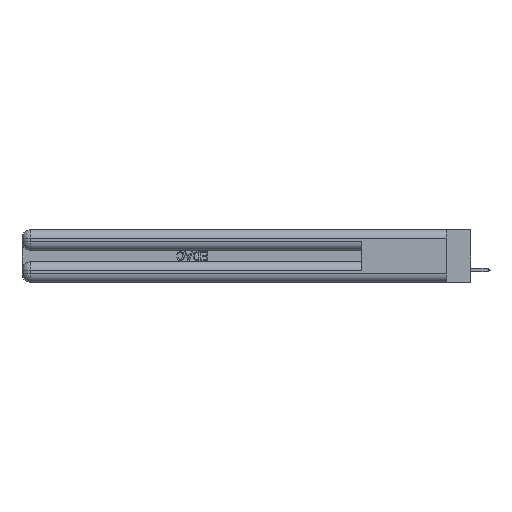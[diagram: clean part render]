
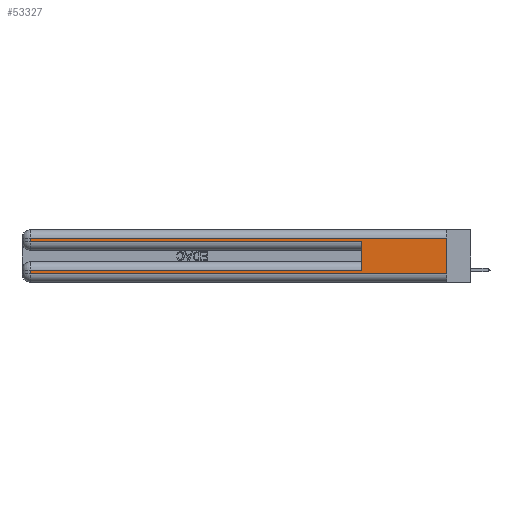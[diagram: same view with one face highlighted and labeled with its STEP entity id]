
A CAD part, left-side view. The second image highlights one B-rep face of the part: STEP entity #53327.
In plain terms, the highlighted planar face has unit normal (-1, 0, 0).
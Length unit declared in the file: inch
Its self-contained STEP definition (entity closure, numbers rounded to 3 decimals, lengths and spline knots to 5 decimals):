
#33 = LINE ( 'NONE', #28466, #30155 ) ;
#564 = LINE ( 'NONE', #40589, #9970 ) ;
#1547 = VECTOR ( 'NONE', #54931, 39.37008 ) ;
#1748 = VERTEX_POINT ( 'NONE', #38078 ) ;
#6576 = DIRECTION ( 'NONE',  ( 1., 0., 0. ) ) ;
#7331 = ORIENTED_EDGE ( 'NONE', *, *, #39463, .F. ) ;
#7527 = LINE ( 'NONE', #45125, #20827 ) ;
#7968 = CARTESIAN_POINT ( 'NONE',  ( 0., 0., 0.285 ) ) ;
#8799 = ORIENTED_EDGE ( 'NONE', *, *, #52723, .F. ) ;
#8872 = EDGE_CURVE ( 'NONE', #46090, #37029, #24621, .T. ) ;
#9970 = VECTOR ( 'NONE', #40776, 39.37008 ) ;
#10214 = ORIENTED_EDGE ( 'NONE', *, *, #16067, .T. ) ;
#11751 = VECTOR ( 'NONE', #34062, 39.37008 ) ;
#11789 = CARTESIAN_POINT ( 'NONE',  ( 0., 2.94, 0.37 ) ) ;
#12263 = CARTESIAN_POINT ( 'NONE',  ( 0., 0., 0.31 ) ) ;
#12292 = ORIENTED_EDGE ( 'NONE', *, *, #22963, .T. ) ;
#14027 = ORIENTED_EDGE ( 'NONE', *, *, #29705, .T. ) ;
#15712 = LINE ( 'NONE', #12263, #48529 ) ;
#15837 = ORIENTED_EDGE ( 'NONE', *, *, #33867, .T. ) ;
#16067 = EDGE_CURVE ( 'NONE', #47234, #22512, #33, .T. ) ;
#16085 = CARTESIAN_POINT ( 'NONE',  ( 0., 2.94, 0.085 ) ) ;
#19209 = ORIENTED_EDGE ( 'NONE', *, *, #8872, .T. ) ;
#19803 = DIRECTION ( 'NONE',  ( 0., 0., -1. ) ) ;
#20521 = DIRECTION ( 'NONE',  ( 0., 0., -1. ) ) ;
#20827 = VECTOR ( 'NONE', #28217, 39.37008 ) ;
#22124 = EDGE_LOOP ( 'NONE', ( #8799, #14027, #19209, #12292, #7331, #49239, #15837, #10214 ) ) ;
#22386 = CARTESIAN_POINT ( 'NONE',  ( 0., 0.6, 0.285 ) ) ;
#22512 = VERTEX_POINT ( 'NONE', #51969 ) ;
#22963 = EDGE_CURVE ( 'NONE', #37029, #35034, #24293, .T. ) ;
#23116 = CARTESIAN_POINT ( 'NONE',  ( 0., 2.94, 0.285 ) ) ;
#24293 = LINE ( 'NONE', #7968, #1547 ) ;
#24302 = EDGE_CURVE ( 'NONE', #1748, #46011, #54484, .T. ) ;
#24621 = LINE ( 'NONE', #11789, #31356 ) ;
#25748 = LINE ( 'NONE', #29728, #11751 ) ;
#27650 = CARTESIAN_POINT ( 'NONE',  ( 0., 0., 0.37 ) ) ;
#28013 = CARTESIAN_POINT ( 'NONE',  ( 0., 0., 0.31 ) ) ;
#28217 = DIRECTION ( 'NONE',  ( 0., 0., 1. ) ) ;
#28279 = DIRECTION ( 'NONE',  ( 0., -1., 0. ) ) ;
#28466 = CARTESIAN_POINT ( 'NONE',  ( 0., 0., 0.06 ) ) ;
#29705 = EDGE_CURVE ( 'NONE', #52740, #46090, #15712, .T. ) ;
#29728 = CARTESIAN_POINT ( 'NONE',  ( 0., 2.94, 0.37 ) ) ;
#30155 = VECTOR ( 'NONE', #28279, 39.37008 ) ;
#31356 = VECTOR ( 'NONE', #20521, 39.37008 ) ;
#32387 = PLANE ( 'NONE',  #39688 ) ;
#33867 = EDGE_CURVE ( 'NONE', #46011, #47234, #25748, .T. ) ;
#34050 = FACE_OUTER_BOUND ( 'NONE', #22124, .T. ) ;
#34062 = DIRECTION ( 'NONE',  ( 0., 0., -1. ) ) ;
#34533 = CARTESIAN_POINT ( 'NONE',  ( 0., 0., 0.085 ) ) ;
#35034 = VERTEX_POINT ( 'NONE', #22386 ) ;
#36406 = CARTESIAN_POINT ( 'NONE',  ( 0., 2.94, 0.06 ) ) ;
#37029 = VERTEX_POINT ( 'NONE', #23116 ) ;
#37785 = VECTOR ( 'NONE', #52323, 39.37008 ) ;
#37914 = DIRECTION ( 'NONE',  ( 0., 1., 0. ) ) ;
#38078 = CARTESIAN_POINT ( 'NONE',  ( 0., 0.6, 0.085 ) ) ;
#39463 = EDGE_CURVE ( 'NONE', #1748, #35034, #7527, .T. ) ;
#39688 = AXIS2_PLACEMENT_3D ( 'NONE', #27650, #6576, #19803 ) ;
#40589 = CARTESIAN_POINT ( 'NONE',  ( 0., 0., 0.37 ) ) ;
#40776 = DIRECTION ( 'NONE',  ( 0., 0., -1. ) ) ;
#42120 = CARTESIAN_POINT ( 'NONE',  ( 0., 2.94, 0.31 ) ) ;
#45125 = CARTESIAN_POINT ( 'NONE',  ( 0., 0.6, 0.145 ) ) ;
#46011 = VERTEX_POINT ( 'NONE', #16085 ) ;
#46090 = VERTEX_POINT ( 'NONE', #42120 ) ;
#47234 = VERTEX_POINT ( 'NONE', #36406 ) ;
#48529 = VECTOR ( 'NONE', #37914, 39.37008 ) ;
#49239 = ORIENTED_EDGE ( 'NONE', *, *, #24302, .T. ) ;
#51969 = CARTESIAN_POINT ( 'NONE',  ( 0., 0., 0.06 ) ) ;
#52323 = DIRECTION ( 'NONE',  ( 0., 1., 0. ) ) ;
#52723 = EDGE_CURVE ( 'NONE', #52740, #22512, #564, .T. ) ;
#52740 = VERTEX_POINT ( 'NONE', #28013 ) ;
#53327 = ADVANCED_FACE ( 'NONE', ( #34050 ), #32387, .F. ) ;
#54484 = LINE ( 'NONE', #34533, #37785 ) ;
#54931 = DIRECTION ( 'NONE',  ( 0., -1., 0. ) ) ;
